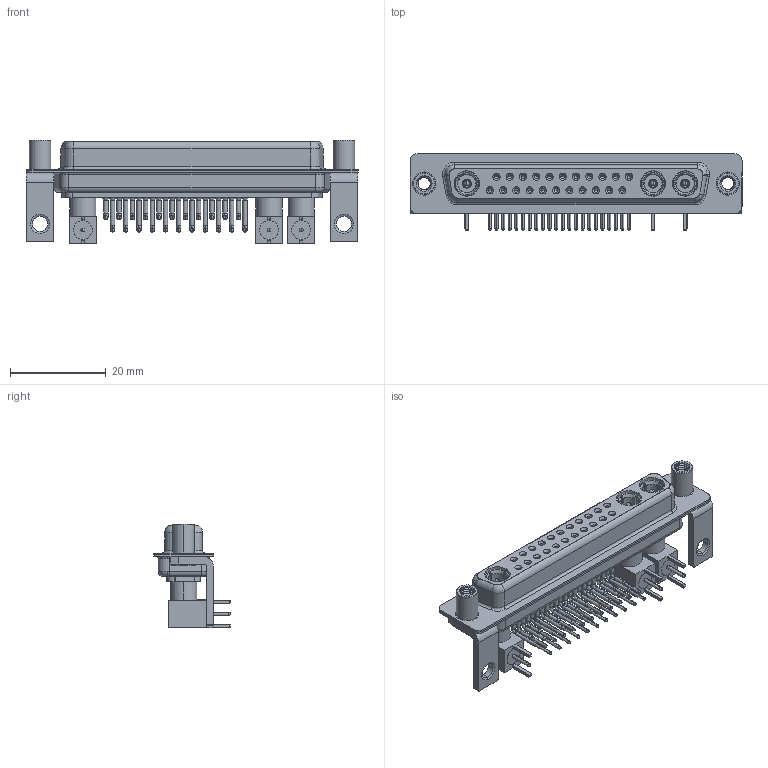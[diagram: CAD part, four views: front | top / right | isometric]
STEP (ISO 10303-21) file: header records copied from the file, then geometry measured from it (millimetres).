
FILE_DESCRIPTION (( 'STEP AP203' ), '1' );
FILE_NAME ('630-25W3640-7TE.STEP', '2022-06-07T09:00:35', ( '' ), ( '' ), 'SwSTEP 2.0', 'SolidWorks 2020', '' );
FILE_SCHEMA (( 'CONFIG_CONTROL_DESIGN' ));
Length unit declared in the file: millimetre
Products named in the file (17): Co-Ax Plug Assy_RA; 630Combo Shell Front_37 Contacts; Pin_RA; 630Combo Housing_25W3; 630Combo Stabilizer Bracket; Insulator RA Pin; Locking Collar; 630-25W3640-7TE; 630Combo Contact Row 1; Co-Ax Plug_RA PC Tail; RA Back Shell; 630Combo Shell Rear_37 Contacts; 630Combo Contact Row 2; Insulator Pin_Straight PC Tail; 630Combo Threaded Standoff_D
Assembly tree (50 placements, depth 3):
  630-25W3640-7TE
    630Combo Housing_25W3
    630Combo Shell Front_37 Contacts
    630Combo Shell Rear_37 Contacts
    630Combo Stabilizer Bracket  x2
    630Combo Threaded Standoff_D  x2
    Co-Ax Plug Assy_RA
      Co-Ax Plug_RA PC Tail
      Insulator Pin_Straight PC Tail
      Pin_RA
      Locking Collar
      RA Back Shell
      Insulator RA Pin
    Co-Ax Plug Assy_RA
      Co-Ax Plug_RA PC Tail
      Insulator Pin_Straight PC Tail
      Pin_RA
      Locking Collar
      RA Back Shell
      Insulator RA Pin
    Co-Ax Plug Assy_RA
      Co-Ax Plug_RA PC Tail
      Insulator Pin_Straight PC Tail
      Pin_RA
      Locking Collar
      RA Back Shell
      Insulator RA Pin
    630Combo Contact Row 1  x11
    630Combo Contact Row 2  x11
Bounding box: 69.4 x 16 x 21.61 mm (x, y, z)
Volume: 6556.7 mm3; surface area: 15504.5 mm2
Topology: 47 solids, 47 shells, 2047 faces, 5128 edges, 3228 vertices
Faces by surface type: cylinder 910, plane 620, cone 333, bspline 97, torus 75, sphere 12
Entity records: 29874 total; most frequent: CARTESIAN_POINT 7053, DIRECTION 4582, ORIENTED_EDGE 3948, EDGE_CURVE 1974, AXIS2_PLACEMENT_3D 1887, VERTEX_POINT 1259, EDGE_LOOP 1013, CIRCLE 1004
